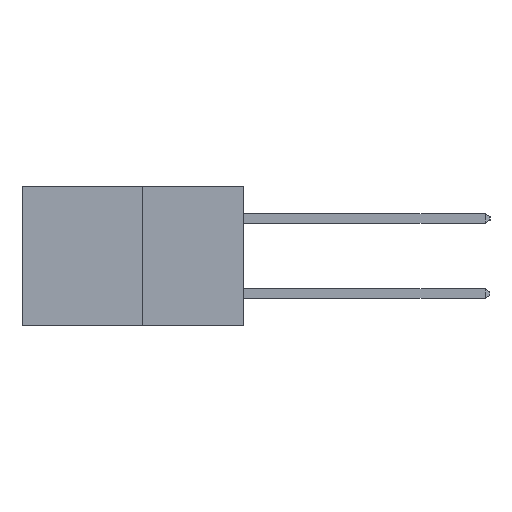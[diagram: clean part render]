
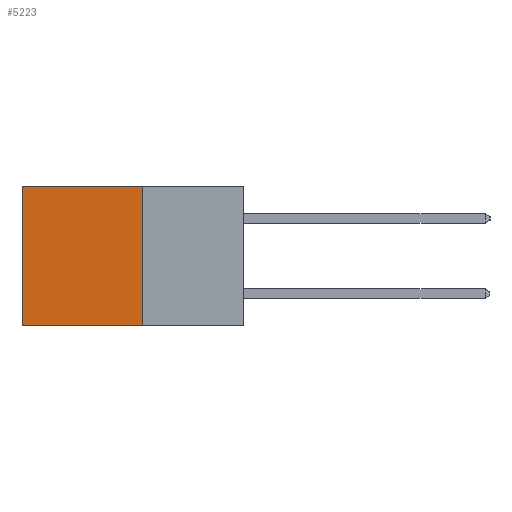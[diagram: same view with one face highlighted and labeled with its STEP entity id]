
A CAD part, left-side view. The second image highlights one B-rep face of the part: STEP entity #5223.
In plain terms, the highlighted planar face has unit normal (-1, 0, 0).
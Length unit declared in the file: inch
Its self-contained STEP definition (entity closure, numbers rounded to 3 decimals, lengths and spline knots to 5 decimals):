
#106 = ORIENTED_EDGE ( 'NONE', *, *, #7474, .F. ) ;
#137 = DIRECTION ( 'NONE',  ( 0., 0., -1. ) ) ;
#425 = FACE_OUTER_BOUND ( 'NONE', #2483, .T. ) ;
#717 = VECTOR ( 'NONE', #137, 39.37008 ) ;
#1686 = EDGE_CURVE ( 'NONE', #1948, #7470, #3700, .T. ) ;
#1948 = VERTEX_POINT ( 'NONE', #2795 ) ;
#2483 = EDGE_LOOP ( 'NONE', ( #7299, #3059, #106, #14010 ) ) ;
#2795 = CARTESIAN_POINT ( 'NONE',  ( 0.277, 0.59, 0. ) ) ;
#3059 = ORIENTED_EDGE ( 'NONE', *, *, #4406, .F. ) ;
#3606 = CARTESIAN_POINT ( 'NONE',  ( 0.277, 0.27, 0. ) ) ;
#3700 = LINE ( 'NONE', #11080, #9473 ) ;
#4124 = EDGE_CURVE ( 'NONE', #6221, #1948, #8759, .T. ) ;
#4406 = EDGE_CURVE ( 'NONE', #14243, #7470, #10847, .T. ) ;
#4630 = CARTESIAN_POINT ( 'NONE',  ( 0.277, 0.27, -0.37 ) ) ;
#5069 = AXIS2_PLACEMENT_3D ( 'NONE', #8509, #8328, #8323 ) ;
#5223 = ADVANCED_FACE ( 'NONE', ( #425 ), #8423, .F. ) ;
#6049 = VECTOR ( 'NONE', #6630, 39.37008 ) ;
#6220 = CARTESIAN_POINT ( 'NONE',  ( 0.277, 0.27, 0. ) ) ;
#6221 = VERTEX_POINT ( 'NONE', #3606 ) ;
#6630 = DIRECTION ( 'NONE',  ( 0., 1., 0. ) ) ;
#7299 = ORIENTED_EDGE ( 'NONE', *, *, #1686, .T. ) ;
#7470 = VERTEX_POINT ( 'NONE', #12636 ) ;
#7474 = EDGE_CURVE ( 'NONE', #6221, #14243, #12839, .T. ) ;
#7838 = VECTOR ( 'NONE', #14358, 39.37008 ) ;
#8323 = DIRECTION ( 'NONE',  ( 0., 0., -1. ) ) ;
#8328 = DIRECTION ( 'NONE',  ( 1., 0., 0. ) ) ;
#8423 = PLANE ( 'NONE',  #5069 ) ;
#8509 = CARTESIAN_POINT ( 'NONE',  ( 0.277, 0.27, -0.37 ) ) ;
#8759 = LINE ( 'NONE', #6220, #6049 ) ;
#9329 = CARTESIAN_POINT ( 'NONE',  ( 0.277, 0.27, -0.37 ) ) ;
#9473 = VECTOR ( 'NONE', #12570, 39.37008 ) ;
#10847 = LINE ( 'NONE', #14551, #7838 ) ;
#11080 = CARTESIAN_POINT ( 'NONE',  ( 0.277, 0.59, -0.37 ) ) ;
#12570 = DIRECTION ( 'NONE',  ( 0., 0., -1. ) ) ;
#12636 = CARTESIAN_POINT ( 'NONE',  ( 0.277, 0.59, -0.37 ) ) ;
#12839 = LINE ( 'NONE', #9329, #717 ) ;
#14010 = ORIENTED_EDGE ( 'NONE', *, *, #4124, .T. ) ;
#14243 = VERTEX_POINT ( 'NONE', #4630 ) ;
#14358 = DIRECTION ( 'NONE',  ( 0., 1., 0. ) ) ;
#14551 = CARTESIAN_POINT ( 'NONE',  ( 0.277, 0.27, -0.37 ) ) ;
